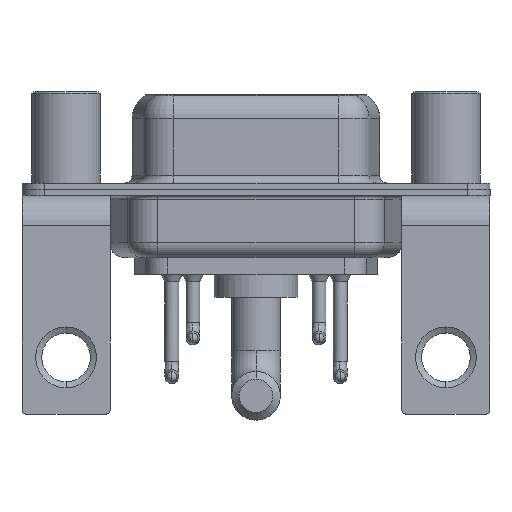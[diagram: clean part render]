
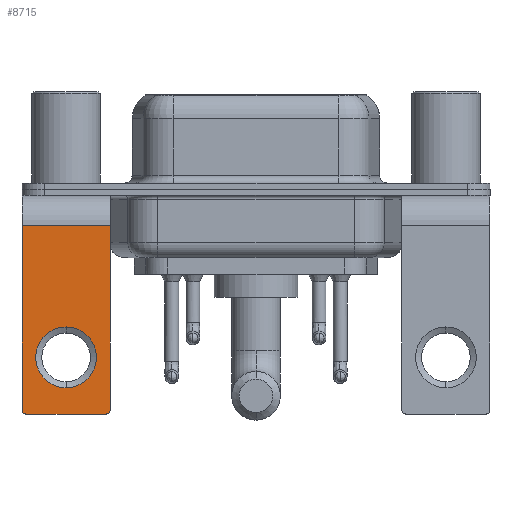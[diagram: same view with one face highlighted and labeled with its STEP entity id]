
A CAD part, front view. The second image highlights one B-rep face of the part: STEP entity #8715.
In plain terms, the highlighted planar face has unit normal (0, -1, 0).
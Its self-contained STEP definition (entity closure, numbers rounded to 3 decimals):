
#49 = LINE ( 'NONE', #10053, #5639 ) ;
#223 = VERTEX_POINT ( 'NONE', #15730 ) ;
#552 = ORIENTED_EDGE ( 'NONE', *, *, #1075, .F. ) ;
#1075 = EDGE_CURVE ( 'NONE', #10394, #223, #49, .T. ) ;
#1100 = CIRCLE ( 'NONE', #2601, 0.25 ) ;
#1271 = VERTEX_POINT ( 'NONE', #7942 ) ;
#1317 = FACE_OUTER_BOUND ( 'NONE', #14364, .T. ) ;
#1380 = CARTESIAN_POINT ( 'NONE',  ( 2.9, -6.25, -14.8 ) ) ;
#1688 = VERTEX_POINT ( 'NONE', #5762 ) ;
#1737 = ORIENTED_EDGE ( 'NONE', *, *, #2238, .T. ) ;
#2022 = CIRCLE ( 'NONE', #2613, 0.25 ) ;
#2238 = EDGE_CURVE ( 'NONE', #1271, #4227, #1100, .T. ) ;
#2459 = EDGE_CURVE ( 'NONE', #1688, #223, #2022, .T. ) ;
#2601 = AXIS2_PLACEMENT_3D ( 'NONE', #10570, #7706, #9233 ) ;
#2613 = AXIS2_PLACEMENT_3D ( 'NONE', #11326, #9605, #17115 ) ;
#2743 = CARTESIAN_POINT ( 'NONE',  ( 2.9, -6.25, -2.4 ) ) ;
#3760 = CARTESIAN_POINT ( 'NONE',  ( 0., -6.25, -9.07 ) ) ;
#4227 = VERTEX_POINT ( 'NONE', #9253 ) ;
#4660 = ORIENTED_EDGE ( 'NONE', *, *, #8008, .F. ) ;
#5404 = ORIENTED_EDGE ( 'NONE', *, *, #15756, .T. ) ;
#5466 = VERTEX_POINT ( 'NONE', #14596 ) ;
#5639 = VECTOR ( 'NONE', #17275, 1000. ) ;
#5718 = AXIS2_PLACEMENT_3D ( 'NONE', #16280, #14752, #17998 ) ;
#5762 = CARTESIAN_POINT ( 'NONE',  ( 2.65, -6.25, -14.8 ) ) ;
#5893 = LINE ( 'NONE', #17296, #13031 ) ;
#6092 = VECTOR ( 'NONE', #7196, 1000. ) ;
#7127 = PLANE ( 'NONE',  #18605 ) ;
#7196 = DIRECTION ( 'NONE',  ( -1., 0., 0. ) ) ;
#7223 = DIRECTION ( 'NONE',  ( 0., 0., -1. ) ) ;
#7231 = VERTEX_POINT ( 'NONE', #3760 ) ;
#7706 = DIRECTION ( 'NONE',  ( 0., -1., 0. ) ) ;
#7942 = CARTESIAN_POINT ( 'NONE',  ( -2.9, -6.25, -14.55 ) ) ;
#7953 = DIRECTION ( 'NONE',  ( 0., 1., 0. ) ) ;
#8008 = EDGE_CURVE ( 'NONE', #1688, #4227, #14418, .T. ) ;
#8213 = ORIENTED_EDGE ( 'NONE', *, *, #12252, .T. ) ;
#8272 = FACE_BOUND ( 'NONE', #18587, .T. ) ;
#8453 = DIRECTION ( 'NONE',  ( 0., 0., 1. ) ) ;
#8715 = ADVANCED_FACE ( 'NONE', ( #8272, #1317 ), #7127, .F. ) ;
#8743 = EDGE_CURVE ( 'NONE', #15536, #1271, #14357, .T. ) ;
#9233 = DIRECTION ( 'NONE',  ( 0., 0., 1. ) ) ;
#9253 = CARTESIAN_POINT ( 'NONE',  ( -2.65, -6.25, -14.8 ) ) ;
#9287 = CARTESIAN_POINT ( 'NONE',  ( 0., -6.25, -11.07 ) ) ;
#9396 = CIRCLE ( 'NONE', #11269, 2. ) ;
#9605 = DIRECTION ( 'NONE',  ( 0., -1., 0. ) ) ;
#10053 = CARTESIAN_POINT ( 'NONE',  ( 2.9, -6.25, -2.4 ) ) ;
#10077 = CARTESIAN_POINT ( 'NONE',  ( -2.9, -6.25, -2.4 ) ) ;
#10394 = VERTEX_POINT ( 'NONE', #11262 ) ;
#10570 = CARTESIAN_POINT ( 'NONE',  ( -2.65, -6.25, -14.55 ) ) ;
#11262 = CARTESIAN_POINT ( 'NONE',  ( 2.9, -6.25, -2.4 ) ) ;
#11269 = AXIS2_PLACEMENT_3D ( 'NONE', #9287, #7953, #12326 ) ;
#11326 = CARTESIAN_POINT ( 'NONE',  ( 2.65, -6.25, -14.55 ) ) ;
#11700 = ORIENTED_EDGE ( 'NONE', *, *, #2459, .T. ) ;
#12093 = CARTESIAN_POINT ( 'NONE',  ( -2.9, -6.25, -2.4 ) ) ;
#12252 = EDGE_CURVE ( 'NONE', #10394, #15536, #5893, .T. ) ;
#12326 = DIRECTION ( 'NONE',  ( 0., 0., 1. ) ) ;
#12829 = VECTOR ( 'NONE', #7223, 1000. ) ;
#13031 = VECTOR ( 'NONE', #14436, 1000. ) ;
#13282 = CIRCLE ( 'NONE', #5718, 2. ) ;
#14312 = ORIENTED_EDGE ( 'NONE', *, *, #8743, .T. ) ;
#14357 = LINE ( 'NONE', #10077, #12829 ) ;
#14364 = EDGE_LOOP ( 'NONE', ( #14312, #1737, #4660, #11700, #552, #8213 ) ) ;
#14418 = LINE ( 'NONE', #1380, #6092 ) ;
#14436 = DIRECTION ( 'NONE',  ( -1., 0., 0. ) ) ;
#14596 = CARTESIAN_POINT ( 'NONE',  ( 0., -6.25, -13.07 ) ) ;
#14752 = DIRECTION ( 'NONE',  ( 0., 1., 0. ) ) ;
#15536 = VERTEX_POINT ( 'NONE', #12093 ) ;
#15730 = CARTESIAN_POINT ( 'NONE',  ( 2.9, -6.25, -14.55 ) ) ;
#15756 = EDGE_CURVE ( 'NONE', #7231, #5466, #13282, .T. ) ;
#16280 = CARTESIAN_POINT ( 'NONE',  ( 0., -6.25, -11.07 ) ) ;
#17115 = DIRECTION ( 'NONE',  ( 0., 0., 1. ) ) ;
#17275 = DIRECTION ( 'NONE',  ( 0., 0., -1. ) ) ;
#17296 = CARTESIAN_POINT ( 'NONE',  ( 2.9, -6.25, -2.4 ) ) ;
#17871 = ORIENTED_EDGE ( 'NONE', *, *, #18551, .T. ) ;
#17998 = DIRECTION ( 'NONE',  ( 0., 0., 1. ) ) ;
#18451 = DIRECTION ( 'NONE',  ( 0., 1., 0. ) ) ;
#18551 = EDGE_CURVE ( 'NONE', #5466, #7231, #9396, .T. ) ;
#18587 = EDGE_LOOP ( 'NONE', ( #17871, #5404 ) ) ;
#18605 = AXIS2_PLACEMENT_3D ( 'NONE', #2743, #18451, #8453 ) ;
